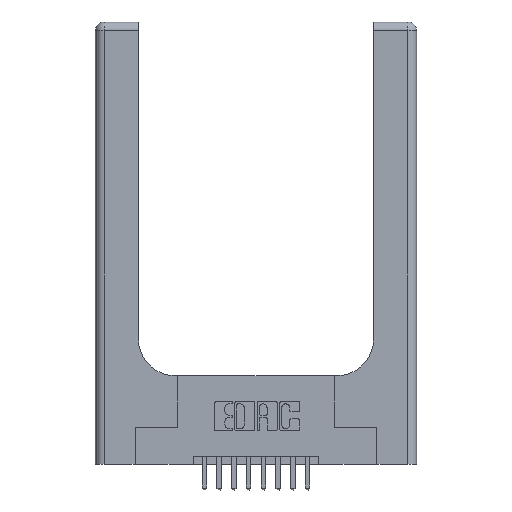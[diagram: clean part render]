
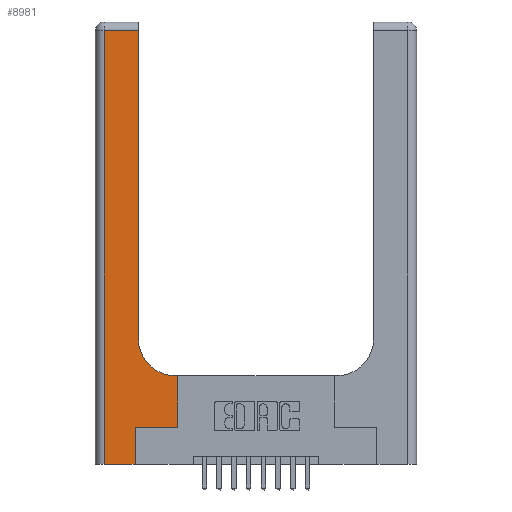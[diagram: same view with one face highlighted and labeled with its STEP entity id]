
A CAD part, top view. The second image highlights one B-rep face of the part: STEP entity #8981.
In plain terms, the highlighted planar face has unit normal (0, 0, 1).
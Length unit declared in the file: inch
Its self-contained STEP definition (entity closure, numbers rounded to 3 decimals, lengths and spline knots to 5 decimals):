
#173 = VERTEX_POINT ( 'NONE', #384 ) ;
#296 = CARTESIAN_POINT ( 'NONE',  ( 0.2915, 0.85, 0.37 ) ) ;
#384 = CARTESIAN_POINT ( 'NONE',  ( 0.5585, 0.25, 0.37 ) ) ;
#401 = ORIENTED_EDGE ( 'NONE', *, *, #2844, .T. ) ;
#958 = CARTESIAN_POINT ( 'NONE',  ( 0., 0., 0.37 ) ) ;
#1116 = EDGE_CURVE ( 'NONE', #2984, #5632, #2864, .T. ) ;
#1312 = EDGE_CURVE ( 'NONE', #10237, #15669, #6781, .T. ) ;
#2137 = ORIENTED_EDGE ( 'NONE', *, *, #1312, .T. ) ;
#2616 = DIRECTION ( 'NONE',  ( 1., 0., 0. ) ) ;
#2774 = EDGE_CURVE ( 'NONE', #173, #10068, #7347, .T. ) ;
#2832 = CARTESIAN_POINT ( 'NONE',  ( 0.269, 0.25, 0.37 ) ) ;
#2839 = LINE ( 'NONE', #4377, #5768 ) ;
#2844 = EDGE_CURVE ( 'NONE', #11908, #6134, #2839, .T. ) ;
#2864 = LINE ( 'NONE', #13540, #12498 ) ;
#2984 = VERTEX_POINT ( 'NONE', #15304 ) ;
#4202 = CARTESIAN_POINT ( 'NONE',  ( 0.06, 0., 0.37 ) ) ;
#4377 = CARTESIAN_POINT ( 'NONE',  ( 0.2915, 3., 0.37 ) ) ;
#4379 = ORIENTED_EDGE ( 'NONE', *, *, #2774, .T. ) ;
#4655 = ORIENTED_EDGE ( 'NONE', *, *, #6559, .T. ) ;
#4763 = DIRECTION ( 'NONE',  ( 0., 1., 0. ) ) ;
#4834 = CARTESIAN_POINT ( 'NONE',  ( 0., 3., 0.37 ) ) ;
#5179 = VECTOR ( 'NONE', #5249, 39.37008 ) ;
#5249 = DIRECTION ( 'NONE',  ( -1., 0., 0. ) ) ;
#5449 = CARTESIAN_POINT ( 'NONE',  ( 0.06, 2.94, 0.37 ) ) ;
#5632 = VERTEX_POINT ( 'NONE', #2832 ) ;
#5768 = VECTOR ( 'NONE', #4763, 39.37008 ) ;
#5793 = VECTOR ( 'NONE', #15885, 39.37008 ) ;
#6100 = DIRECTION ( 'NONE',  ( 0., 0., -1. ) ) ;
#6134 = VERTEX_POINT ( 'NONE', #8794 ) ;
#6361 = CARTESIAN_POINT ( 'NONE',  ( 0.5415, 0.85, 0.37 ) ) ;
#6410 = VECTOR ( 'NONE', #2616, 39.37008 ) ;
#6559 = EDGE_CURVE ( 'NONE', #5632, #173, #13107, .T. ) ;
#6781 = LINE ( 'NONE', #11884, #7170 ) ;
#7170 = VECTOR ( 'NONE', #11883, 39.37008 ) ;
#7347 = LINE ( 'NONE', #8837, #9885 ) ;
#7642 = DIRECTION ( 'NONE',  ( 1., 0., 0. ) ) ;
#8017 = VERTEX_POINT ( 'NONE', #14847 ) ;
#8511 = CARTESIAN_POINT ( 'NONE',  ( 0.5585, 0.6, 0.37 ) ) ;
#8570 = DIRECTION ( 'NONE',  ( 0., 1., 0. ) ) ;
#8794 = CARTESIAN_POINT ( 'NONE',  ( 0.2915, 2.94, 0.37 ) ) ;
#8837 = CARTESIAN_POINT ( 'NONE',  ( 0.5585, 0.25, 0.37 ) ) ;
#8981 = ADVANCED_FACE ( 'NONE', ( #14922 ), #12392, .F. ) ;
#9126 = VECTOR ( 'NONE', #13075, 39.37008 ) ;
#9329 = LINE ( 'NONE', #12803, #5179 ) ;
#9885 = VECTOR ( 'NONE', #8570, 39.37008 ) ;
#9977 = ORIENTED_EDGE ( 'NONE', *, *, #14909, .T. ) ;
#10068 = VERTEX_POINT ( 'NONE', #8511 ) ;
#10237 = VERTEX_POINT ( 'NONE', #5449 ) ;
#10561 = CARTESIAN_POINT ( 'NONE',  ( 0., 2.94, 0.37 ) ) ;
#10673 = EDGE_LOOP ( 'NONE', ( #401, #14184, #2137, #14886, #12442, #4655, #4379, #15503, #9977 ) ) ;
#11430 = CARTESIAN_POINT ( 'NONE',  ( 0.269, 0.25, 0.37 ) ) ;
#11883 = DIRECTION ( 'NONE',  ( 0., -1., 0. ) ) ;
#11884 = CARTESIAN_POINT ( 'NONE',  ( 0.06, 3., 0.37 ) ) ;
#11908 = VERTEX_POINT ( 'NONE', #296 ) ;
#12392 = PLANE ( 'NONE',  #13197 ) ;
#12442 = ORIENTED_EDGE ( 'NONE', *, *, #1116, .T. ) ;
#12498 = VECTOR ( 'NONE', #13701, 39.37008 ) ;
#12803 = CARTESIAN_POINT ( 'NONE',  ( 0.2915, 0.6, 0.37 ) ) ;
#12877 = LINE ( 'NONE', #958, #5793 ) ;
#13075 = DIRECTION ( 'NONE',  ( -1., 0., 0. ) ) ;
#13107 = LINE ( 'NONE', #11430, #6410 ) ;
#13197 = AXIS2_PLACEMENT_3D ( 'NONE', #4834, #6100, #14838 ) ;
#13540 = CARTESIAN_POINT ( 'NONE',  ( 0.269, 0., 0.37 ) ) ;
#13701 = DIRECTION ( 'NONE',  ( 0., 1., 0. ) ) ;
#14184 = ORIENTED_EDGE ( 'NONE', *, *, #15102, .T. ) ;
#14672 = EDGE_CURVE ( 'NONE', #15669, #2984, #12877, .T. ) ;
#14838 = DIRECTION ( 'NONE',  ( -1., 0., 0. ) ) ;
#14847 = CARTESIAN_POINT ( 'NONE',  ( 0.5415, 0.6, 0.37 ) ) ;
#14886 = ORIENTED_EDGE ( 'NONE', *, *, #14672, .T. ) ;
#14909 = EDGE_CURVE ( 'NONE', #8017, #11908, #15532, .T. ) ;
#14922 = FACE_OUTER_BOUND ( 'NONE', #10673, .T. ) ;
#14987 = EDGE_CURVE ( 'NONE', #10068, #8017, #9329, .T. ) ;
#15059 = AXIS2_PLACEMENT_3D ( 'NONE', #6361, #15085, #7642 ) ;
#15085 = DIRECTION ( 'NONE',  ( 0., 0., -1. ) ) ;
#15102 = EDGE_CURVE ( 'NONE', #6134, #10237, #15702, .T. ) ;
#15304 = CARTESIAN_POINT ( 'NONE',  ( 0.269, 0., 0.37 ) ) ;
#15503 = ORIENTED_EDGE ( 'NONE', *, *, #14987, .T. ) ;
#15532 = CIRCLE ( 'NONE', #15059, 0.25 ) ;
#15669 = VERTEX_POINT ( 'NONE', #4202 ) ;
#15702 = LINE ( 'NONE', #10561, #9126 ) ;
#15885 = DIRECTION ( 'NONE',  ( 1., 0., 0. ) ) ;
